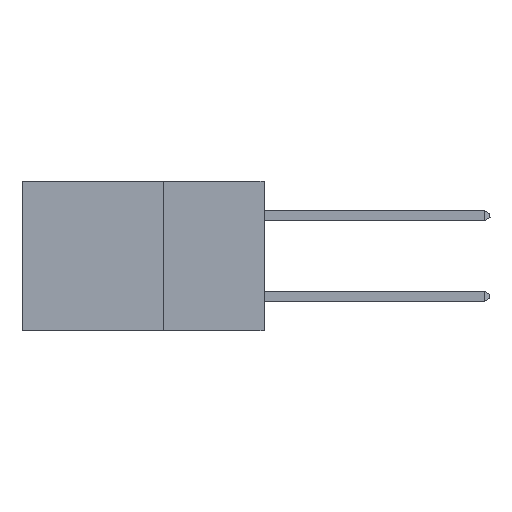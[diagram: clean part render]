
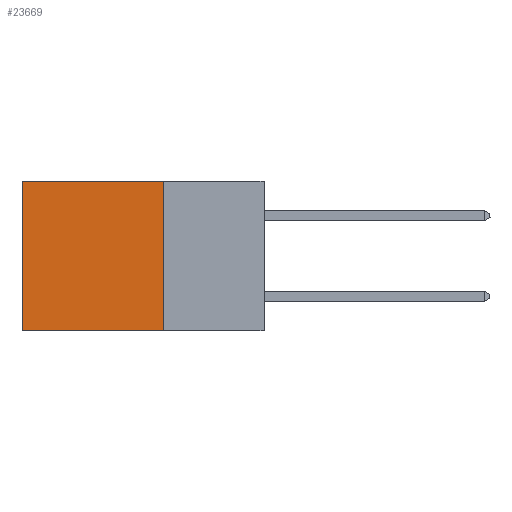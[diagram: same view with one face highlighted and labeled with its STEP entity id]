
A CAD part, left-side view. The second image highlights one B-rep face of the part: STEP entity #23669.
In plain terms, the highlighted planar face has unit normal (-1, 0, 0).
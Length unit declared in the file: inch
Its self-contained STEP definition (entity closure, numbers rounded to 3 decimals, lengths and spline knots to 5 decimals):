
#375 = DIRECTION ( 'NONE',  ( 0., 0., -1. ) ) ;
#488 = DIRECTION ( 'NONE',  ( 0., 0., -1. ) ) ;
#625 = VECTOR ( 'NONE', #2824, 39.37008 ) ;
#1784 = CARTESIAN_POINT ( 'NONE',  ( 0.298, 0.25, -0.37 ) ) ;
#2018 = DIRECTION ( 'NONE',  ( 1., 0., 0. ) ) ;
#2642 = VECTOR ( 'NONE', #488, 39.37008 ) ;
#2824 = DIRECTION ( 'NONE',  ( 0., 0., -1. ) ) ;
#2940 = VERTEX_POINT ( 'NONE', #23046 ) ;
#4420 = ORIENTED_EDGE ( 'NONE', *, *, #14416, .T. ) ;
#6309 = LINE ( 'NONE', #1784, #21056 ) ;
#6754 = CARTESIAN_POINT ( 'NONE',  ( 0.298, 0.25, 0. ) ) ;
#6959 = EDGE_CURVE ( 'NONE', #2940, #16918, #6309, .T. ) ;
#8401 = ORIENTED_EDGE ( 'NONE', *, *, #17059, .T. ) ;
#10064 = VERTEX_POINT ( 'NONE', #6754 ) ;
#11111 = EDGE_LOOP ( 'NONE', ( #8401, #17833, #16537, #4420 ) ) ;
#11248 = VECTOR ( 'NONE', #13636, 39.37008 ) ;
#11428 = FACE_OUTER_BOUND ( 'NONE', #11111, .T. ) ;
#11675 = DIRECTION ( 'NONE',  ( 0., 1., 0. ) ) ;
#12230 = AXIS2_PLACEMENT_3D ( 'NONE', #13791, #2018, #375 ) ;
#13163 = VERTEX_POINT ( 'NONE', #20886 ) ;
#13636 = DIRECTION ( 'NONE',  ( 0., 1., 0. ) ) ;
#13717 = CARTESIAN_POINT ( 'NONE',  ( 0.298, 0.25, 0. ) ) ;
#13791 = CARTESIAN_POINT ( 'NONE',  ( 0.298, 0.25, 0. ) ) ;
#14202 = EDGE_CURVE ( 'NONE', #10064, #2940, #24813, .T. ) ;
#14416 = EDGE_CURVE ( 'NONE', #10064, #13163, #14956, .T. ) ;
#14611 = CARTESIAN_POINT ( 'NONE',  ( 0.298, 0.6, 0. ) ) ;
#14956 = LINE ( 'NONE', #13717, #11248 ) ;
#16537 = ORIENTED_EDGE ( 'NONE', *, *, #14202, .F. ) ;
#16918 = VERTEX_POINT ( 'NONE', #23436 ) ;
#17059 = EDGE_CURVE ( 'NONE', #13163, #16918, #24355, .T. ) ;
#17833 = ORIENTED_EDGE ( 'NONE', *, *, #6959, .F. ) ;
#20886 = CARTESIAN_POINT ( 'NONE',  ( 0.298, 0.6, 0. ) ) ;
#21056 = VECTOR ( 'NONE', #11675, 39.37008 ) ;
#21613 = PLANE ( 'NONE',  #12230 ) ;
#22093 = CARTESIAN_POINT ( 'NONE',  ( 0.298, 0.25, 0. ) ) ;
#23046 = CARTESIAN_POINT ( 'NONE',  ( 0.298, 0.25, -0.37 ) ) ;
#23436 = CARTESIAN_POINT ( 'NONE',  ( 0.298, 0.6, -0.37 ) ) ;
#23669 = ADVANCED_FACE ( 'NONE', ( #11428 ), #21613, .F. ) ;
#24355 = LINE ( 'NONE', #14611, #625 ) ;
#24813 = LINE ( 'NONE', #22093, #2642 ) ;
